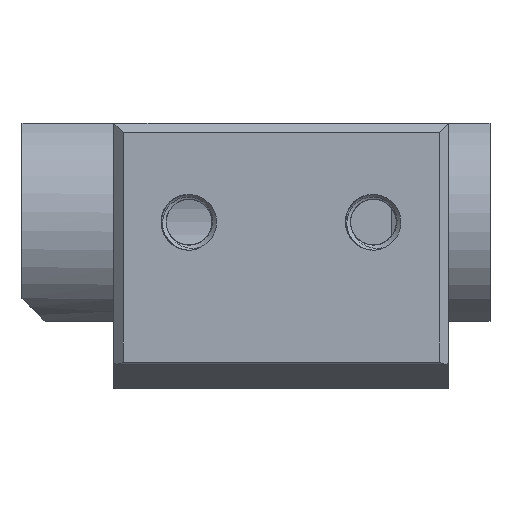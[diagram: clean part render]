
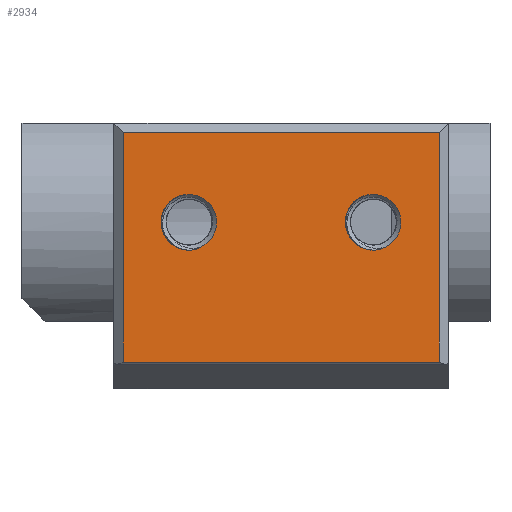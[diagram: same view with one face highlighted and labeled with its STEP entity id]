
A CAD part, front view. The second image highlights one B-rep face of the part: STEP entity #2934.
In plain terms, the highlighted planar face has unit normal (0, -1, 0).
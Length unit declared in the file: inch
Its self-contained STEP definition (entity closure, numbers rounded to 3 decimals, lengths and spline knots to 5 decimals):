
#20=FACE_BOUND('',#374,.T.);
#21=FACE_BOUND('',#375,.T.);
#43=PLANE('',#3118);
#114=CIRCLE('',#3056,0.06075);
#115=CIRCLE('',#3069,0.06075);
#117=CIRCLE('',#3081,0.05978);
#119=CIRCLE('',#3095,0.05978);
#120=CIRCLE('',#3097,0.05978);
#121=CIRCLE('',#3100,0.05978);
#214=FACE_OUTER_BOUND('',#373,.T.);
#373=EDGE_LOOP('',(#2194,#2195,#2196,#2197));
#374=EDGE_LOOP('',(#2198,#2199,#2200,#2201,#2202));
#375=EDGE_LOOP('',(#2203,#2204,#2205,#2206,#2207));
#579=B_SPLINE_CURVE_WITH_KNOTS('',3,(#5836,#5837,#5838,#5839),
 .UNSPECIFIED.,.F.,.F.,(4,4),(0.,0.02741),.UNSPECIFIED.);
#588=B_SPLINE_CURVE_WITH_KNOTS('',3,(#6339,#6340,#6341,#6342),
 .UNSPECIFIED.,.F.,.F.,(4,4),(0.,0.02741),.UNSPECIFIED.);
#594=B_SPLINE_CURVE_WITH_KNOTS('',3,(#6509,#6510,#6511,#6512,#6513,#6514,
#6515),.UNSPECIFIED.,.F.,.F.,(4,3,4),(0.25789,0.2801,
0.28514),.UNSPECIFIED.);
#595=B_SPLINE_CURVE_WITH_KNOTS('',3,(#6516,#6517,#6518,#6519,#6520,#6521,
#6522),.UNSPECIFIED.,.F.,.F.,(4,3,4),(0.25789,0.28176,
0.28514),.UNSPECIFIED.);
#728=LINE('',#6461,#960);
#730=LINE('',#6467,#962);
#733=LINE('',#6473,#965);
#736=LINE('',#6480,#968);
#960=VECTOR('',#3421,0.3937);
#962=VECTOR('',#3427,0.3937);
#965=VECTOR('',#3432,0.3937);
#968=VECTOR('',#3439,0.3937);
#1151=VERTEX_POINT('',#4057);
#1152=VERTEX_POINT('',#4063);
#1179=VERTEX_POINT('',#4343);
#1180=VERTEX_POINT('',#4349);
#1203=VERTEX_POINT('',#4778);
#1205=VERTEX_POINT('',#4781);
#1232=VERTEX_POINT('',#5335);
#1234=VERTEX_POINT('',#5338);
#1235=VERTEX_POINT('',#5442);
#1238=VERTEX_POINT('',#5990);
#1262=VERTEX_POINT('',#6458);
#1263=VERTEX_POINT('',#6460);
#1265=VERTEX_POINT('',#6466);
#1267=VERTEX_POINT('',#6472);
#1460=EDGE_CURVE('',#1152,#1151,#114,.T.);
#1498=EDGE_CURVE('',#1180,#1179,#115,.T.);
#1530=EDGE_CURVE('',#1203,#1205,#117,.T.);
#1568=EDGE_CURVE('',#1232,#1234,#119,.T.);
#1572=EDGE_CURVE('',#1235,#1232,#120,.T.);
#1575=EDGE_CURVE('',#1179,#1234,#579,.T.);
#1582=EDGE_CURVE('',#1238,#1203,#121,.T.);
#1585=EDGE_CURVE('',#1151,#1205,#588,.T.);
#1613=EDGE_CURVE('',#1262,#1263,#728,.T.);
#1616=EDGE_CURVE('',#1265,#1262,#730,.T.);
#1619=EDGE_CURVE('',#1267,#1265,#733,.T.);
#1623=EDGE_CURVE('',#1263,#1267,#736,.T.);
#1638=EDGE_CURVE('',#1235,#1180,#594,.T.);
#1639=EDGE_CURVE('',#1238,#1152,#595,.T.);
#2194=ORIENTED_EDGE('',*,*,#1613,.F.);
#2195=ORIENTED_EDGE('',*,*,#1616,.F.);
#2196=ORIENTED_EDGE('',*,*,#1619,.F.);
#2197=ORIENTED_EDGE('',*,*,#1623,.F.);
#2198=ORIENTED_EDGE('',*,*,#1572,.F.);
#2199=ORIENTED_EDGE('',*,*,#1638,.T.);
#2200=ORIENTED_EDGE('',*,*,#1498,.T.);
#2201=ORIENTED_EDGE('',*,*,#1575,.T.);
#2202=ORIENTED_EDGE('',*,*,#1568,.F.);
#2203=ORIENTED_EDGE('',*,*,#1582,.F.);
#2204=ORIENTED_EDGE('',*,*,#1639,.T.);
#2205=ORIENTED_EDGE('',*,*,#1460,.T.);
#2206=ORIENTED_EDGE('',*,*,#1585,.T.);
#2207=ORIENTED_EDGE('',*,*,#1530,.F.);
#2934=ADVANCED_FACE('',(#214,#20,#21),#43,.T.);
#3056=AXIS2_PLACEMENT_3D('',#4064,#3262,#3263);
#3069=AXIS2_PLACEMENT_3D('',#4350,#3300,#3301);
#3081=AXIS2_PLACEMENT_3D('',#4782,#3334,#3335);
#3095=AXIS2_PLACEMENT_3D('',#5339,#3374,#3375);
#3097=AXIS2_PLACEMENT_3D('',#5471,#3378,#3379);
#3100=AXIS2_PLACEMENT_3D('',#6019,#3384,#3385);
#3118=AXIS2_PLACEMENT_3D('',#6508,#3460,#3461);
#3262=DIRECTION('center_axis',(0.,1.,0.));
#3263=DIRECTION('ref_axis',(1.,0.,0.));
#3300=DIRECTION('center_axis',(0.,1.,0.));
#3301=DIRECTION('ref_axis',(1.,0.,0.));
#3334=DIRECTION('center_axis',(0.,-1.,0.));
#3335=DIRECTION('ref_axis',(1.,0.,0.));
#3374=DIRECTION('center_axis',(0.,-1.,0.));
#3375=DIRECTION('ref_axis',(1.,0.,0.));
#3378=DIRECTION('center_axis',(0.,-1.,0.));
#3379=DIRECTION('ref_axis',(1.,0.,0.));
#3384=DIRECTION('center_axis',(0.,-1.,0.));
#3385=DIRECTION('ref_axis',(1.,0.,0.));
#3421=DIRECTION('',(0.,0.,-1.));
#3427=DIRECTION('',(1.,0.,0.));
#3432=DIRECTION('',(0.,0.,1.));
#3439=DIRECTION('',(-1.,0.,0.));
#3460=DIRECTION('center_axis',(0.,-1.,0.));
#3461=DIRECTION('ref_axis',(0.,0.,1.));
#4057=CARTESIAN_POINT('',(-0.21569,-2.36136,0.12131));
#4063=CARTESIAN_POINT('',(-0.18428,-2.36136,0.12121));
#4064=CARTESIAN_POINT('Origin',(-0.2,-2.36136,0.18));
#4343=CARTESIAN_POINT('',(0.18431,-2.36136,0.12131));
#4349=CARTESIAN_POINT('',(0.21573,-2.36136,0.12121));
#4350=CARTESIAN_POINT('Origin',(0.2,-2.36136,0.18));
#4778=CARTESIAN_POINT('',(-0.25978,-2.36136,0.18));
#4781=CARTESIAN_POINT('',(-0.22541,-2.36136,0.12589));
#4782=CARTESIAN_POINT('Origin',(-0.2,-2.36136,0.18));
#5335=CARTESIAN_POINT('',(0.14022,-2.36136,0.18));
#5338=CARTESIAN_POINT('',(0.17459,-2.36136,0.12589));
#5339=CARTESIAN_POINT('Origin',(0.2,-2.36136,0.18));
#5442=CARTESIAN_POINT('',(0.22541,-2.36136,0.12589));
#5471=CARTESIAN_POINT('Origin',(0.2,-2.36136,0.18));
#5836=CARTESIAN_POINT('Ctrl Pts',(0.18431,-2.36136,0.12131));
#5837=CARTESIAN_POINT('Ctrl Pts',(0.18093,-2.36136,0.12255));
#5838=CARTESIAN_POINT('Ctrl Pts',(0.17769,-2.36136,0.1241));
#5839=CARTESIAN_POINT('Ctrl Pts',(0.17461,-2.36136,0.12593));
#5990=CARTESIAN_POINT('',(-0.17459,-2.36136,0.12589));
#6019=CARTESIAN_POINT('Origin',(-0.2,-2.36136,0.18));
#6339=CARTESIAN_POINT('Ctrl Pts',(-0.21569,-2.36136,
0.12131));
#6340=CARTESIAN_POINT('Ctrl Pts',(-0.21907,-2.36136,
0.12255));
#6341=CARTESIAN_POINT('Ctrl Pts',(-0.22231,-2.36136,
0.1241));
#6342=CARTESIAN_POINT('Ctrl Pts',(-0.22539,-2.36136,
0.12593));
#6458=CARTESIAN_POINT('',(0.343,-2.36136,0.375));
#6460=CARTESIAN_POINT('',(0.343,-2.36136,-0.12364));
#6461=CARTESIAN_POINT('',(0.343,-2.36136,-1.08057));
#6466=CARTESIAN_POINT('',(-0.343,-2.36136,0.375));
#6467=CARTESIAN_POINT('',(-0.0765,-2.36136,0.375));
#6472=CARTESIAN_POINT('',(-0.343,-2.36136,-0.12364));
#6473=CARTESIAN_POINT('',(-0.343,-2.36136,-1.08057));
#6480=CARTESIAN_POINT('',(-0.33,-2.36136,-0.12364));
#6508=CARTESIAN_POINT('Origin',(-0.363,-2.36136,-0.14364));
#6509=CARTESIAN_POINT('Ctrl Pts',(0.22539,-2.36136,0.12582));
#6510=CARTESIAN_POINT('Ctrl Pts',(0.22289,-2.36136,0.12432));
#6511=CARTESIAN_POINT('Ctrl Pts',(0.22028,-2.36136,0.12301));
#6512=CARTESIAN_POINT('Ctrl Pts',(0.21758,-2.36136,0.12192));
#6513=CARTESIAN_POINT('Ctrl Pts',(0.21697,-2.36136,0.12168));
#6514=CARTESIAN_POINT('Ctrl Pts',(0.21635,-2.36136,0.12144));
#6515=CARTESIAN_POINT('Ctrl Pts',(0.21573,-2.36136,0.12121));
#6516=CARTESIAN_POINT('Ctrl Pts',(-0.17461,-2.36136,
0.12582));
#6517=CARTESIAN_POINT('Ctrl Pts',(-0.17731,-2.36136,
0.12421));
#6518=CARTESIAN_POINT('Ctrl Pts',(-0.18012,-2.36136,
0.12282));
#6519=CARTESIAN_POINT('Ctrl Pts',(-0.18303,-2.36136,
0.12168));
#6520=CARTESIAN_POINT('Ctrl Pts',(-0.18344,-2.36136,
0.12152));
#6521=CARTESIAN_POINT('Ctrl Pts',(-0.18386,-2.36136,
0.12136));
#6522=CARTESIAN_POINT('Ctrl Pts',(-0.18428,-2.36136,
0.12121));
